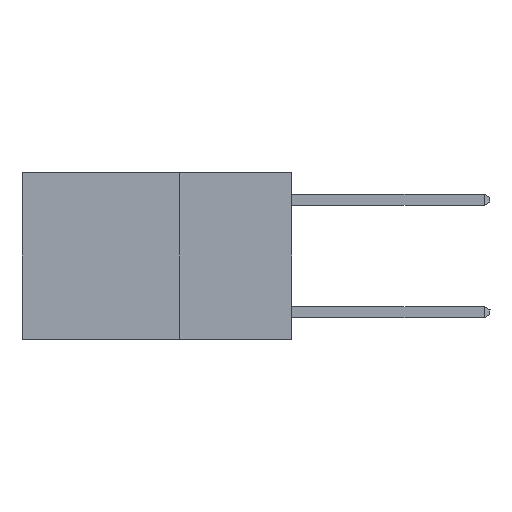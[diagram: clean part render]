
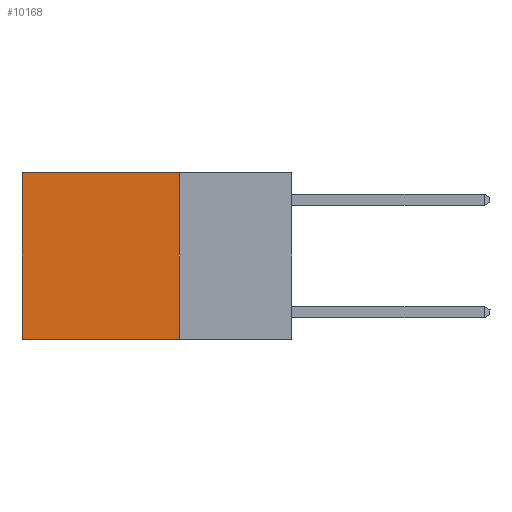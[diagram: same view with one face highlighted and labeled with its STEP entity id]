
A CAD part, left-side view. The second image highlights one B-rep face of the part: STEP entity #10168.
In plain terms, the highlighted planar face has unit normal (-1, 0, 0).
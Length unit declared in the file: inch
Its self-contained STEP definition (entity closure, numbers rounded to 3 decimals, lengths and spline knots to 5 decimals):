
#602 = CARTESIAN_POINT ( 'NONE',  ( 0.2625, 0.6, 0. ) ) ;
#1363 = VECTOR ( 'NONE', #3064, 39.37008 ) ;
#1375 = CARTESIAN_POINT ( 'NONE',  ( 0.2625, 0.25, -0.37 ) ) ;
#1394 = DIRECTION ( 'NONE',  ( 0., 0., -1. ) ) ;
#1524 = VERTEX_POINT ( 'NONE', #2810 ) ;
#1750 = AXIS2_PLACEMENT_3D ( 'NONE', #5811, #6691, #1394 ) ;
#2214 = LINE ( 'NONE', #2378, #11230 ) ;
#2267 = VERTEX_POINT ( 'NONE', #3844 ) ;
#2378 = CARTESIAN_POINT ( 'NONE',  ( 0.2625, 0.25, 0. ) ) ;
#2810 = CARTESIAN_POINT ( 'NONE',  ( 0.2625, 0.6, -0.37 ) ) ;
#2869 = ORIENTED_EDGE ( 'NONE', *, *, #4272, .T. ) ;
#3064 = DIRECTION ( 'NONE',  ( 0., 1., 0. ) ) ;
#3134 = VECTOR ( 'NONE', #5393, 39.37008 ) ;
#3508 = LINE ( 'NONE', #602, #5578 ) ;
#3844 = CARTESIAN_POINT ( 'NONE',  ( 0.2625, 0.6, 0. ) ) ;
#4272 = EDGE_CURVE ( 'NONE', #2267, #1524, #3508, .T. ) ;
#5192 = LINE ( 'NONE', #10614, #3134 ) ;
#5393 = DIRECTION ( 'NONE',  ( 0., 0., -1. ) ) ;
#5578 = VECTOR ( 'NONE', #5916, 39.37008 ) ;
#5811 = CARTESIAN_POINT ( 'NONE',  ( 0.2625, 0.25, 0. ) ) ;
#5916 = DIRECTION ( 'NONE',  ( 0., 0., -1. ) ) ;
#6164 = VERTEX_POINT ( 'NONE', #8024 ) ;
#6691 = DIRECTION ( 'NONE',  ( 1., 0., 0. ) ) ;
#7129 = ORIENTED_EDGE ( 'NONE', *, *, #7583, .F. ) ;
#7461 = CARTESIAN_POINT ( 'NONE',  ( 0.2625, 0.25, -0.37 ) ) ;
#7583 = EDGE_CURVE ( 'NONE', #9556, #1524, #8393, .T. ) ;
#8024 = CARTESIAN_POINT ( 'NONE',  ( 0.2625, 0.25, 0. ) ) ;
#8161 = FACE_OUTER_BOUND ( 'NONE', #8908, .T. ) ;
#8393 = LINE ( 'NONE', #7461, #1363 ) ;
#8546 = ORIENTED_EDGE ( 'NONE', *, *, #8593, .F. ) ;
#8593 = EDGE_CURVE ( 'NONE', #6164, #9556, #5192, .T. ) ;
#8908 = EDGE_LOOP ( 'NONE', ( #2869, #7129, #8546, #11245 ) ) ;
#9413 = DIRECTION ( 'NONE',  ( 0., 1., 0. ) ) ;
#9556 = VERTEX_POINT ( 'NONE', #1375 ) ;
#10168 = ADVANCED_FACE ( 'NONE', ( #8161 ), #11001, .F. ) ;
#10614 = CARTESIAN_POINT ( 'NONE',  ( 0.2625, 0.25, 0. ) ) ;
#10907 = EDGE_CURVE ( 'NONE', #6164, #2267, #2214, .T. ) ;
#11001 = PLANE ( 'NONE',  #1750 ) ;
#11230 = VECTOR ( 'NONE', #9413, 39.37008 ) ;
#11245 = ORIENTED_EDGE ( 'NONE', *, *, #10907, .T. ) ;
